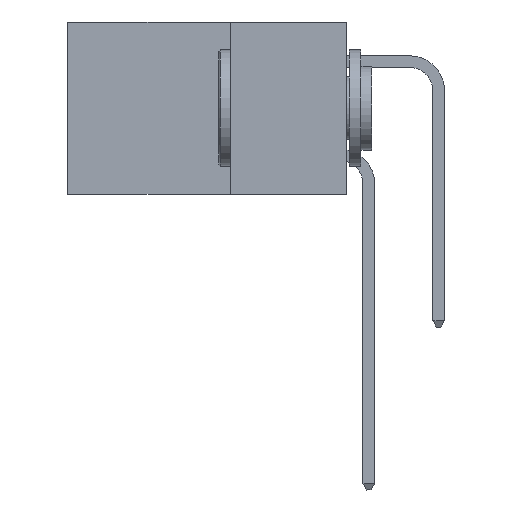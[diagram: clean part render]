
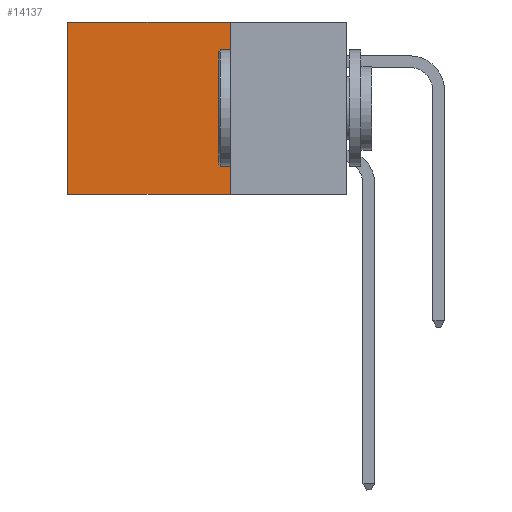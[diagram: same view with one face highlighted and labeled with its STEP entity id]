
A CAD part, left-side view. The second image highlights one B-rep face of the part: STEP entity #14137.
In plain terms, the highlighted planar face has unit normal (-1, 0, 0).
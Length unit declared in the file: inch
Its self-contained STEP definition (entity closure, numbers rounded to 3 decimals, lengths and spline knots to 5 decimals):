
#123 = ORIENTED_EDGE ( 'NONE', *, *, #8447, .T. ) ;
#1247 = VERTEX_POINT ( 'NONE', #9302 ) ;
#1820 = PLANE ( 'NONE',  #14591 ) ;
#2157 = VECTOR ( 'NONE', #8303, 39.37008 ) ;
#2191 = CARTESIAN_POINT ( 'NONE',  ( 0.2875, 0.25, 0. ) ) ;
#2206 = EDGE_LOOP ( 'NONE', ( #123, #6674, #12758, #3878 ) ) ;
#2553 = DIRECTION ( 'NONE',  ( 0., 1., 0. ) ) ;
#3021 = EDGE_CURVE ( 'NONE', #1247, #14370, #9926, .T. ) ;
#3025 = CARTESIAN_POINT ( 'NONE',  ( 0.2875, 0.25, 0. ) ) ;
#3090 = DIRECTION ( 'NONE',  ( 1., 0., 0. ) ) ;
#3215 = LINE ( 'NONE', #9040, #14987 ) ;
#3436 = DIRECTION ( 'NONE',  ( 0., 0., -1. ) ) ;
#3479 = CARTESIAN_POINT ( 'NONE',  ( 0.2875, 0.6, 0. ) ) ;
#3878 = ORIENTED_EDGE ( 'NONE', *, *, #3021, .T. ) ;
#4125 = CARTESIAN_POINT ( 'NONE',  ( 0.2875, 0.25, -0.37 ) ) ;
#5371 = LINE ( 'NONE', #5899, #2157 ) ;
#5899 = CARTESIAN_POINT ( 'NONE',  ( 0.2875, 0.25, -0.37 ) ) ;
#6674 = ORIENTED_EDGE ( 'NONE', *, *, #14986, .F. ) ;
#6804 = CARTESIAN_POINT ( 'NONE',  ( 0.2875, 0.6, -0.37 ) ) ;
#8209 = VECTOR ( 'NONE', #3436, 39.37008 ) ;
#8303 = DIRECTION ( 'NONE',  ( 0., 1., 0. ) ) ;
#8447 = EDGE_CURVE ( 'NONE', #14370, #14822, #3215, .T. ) ;
#8562 = LINE ( 'NONE', #2191, #8209 ) ;
#9000 = CARTESIAN_POINT ( 'NONE',  ( 0.2875, 0.25, 0. ) ) ;
#9040 = CARTESIAN_POINT ( 'NONE',  ( 0.2875, 0.6, 0. ) ) ;
#9302 = CARTESIAN_POINT ( 'NONE',  ( 0.2875, 0.25, 0. ) ) ;
#9543 = VECTOR ( 'NONE', #2553, 39.37008 ) ;
#9926 = LINE ( 'NONE', #3025, #9543 ) ;
#9983 = EDGE_CURVE ( 'NONE', #1247, #13060, #8562, .T. ) ;
#11287 = DIRECTION ( 'NONE',  ( 0., 0., -1. ) ) ;
#12415 = DIRECTION ( 'NONE',  ( 0., 0., -1. ) ) ;
#12758 = ORIENTED_EDGE ( 'NONE', *, *, #9983, .F. ) ;
#13060 = VERTEX_POINT ( 'NONE', #4125 ) ;
#13790 = FACE_OUTER_BOUND ( 'NONE', #2206, .T. ) ;
#14137 = ADVANCED_FACE ( 'NONE', ( #13790 ), #1820, .F. ) ;
#14370 = VERTEX_POINT ( 'NONE', #3479 ) ;
#14591 = AXIS2_PLACEMENT_3D ( 'NONE', #9000, #3090, #11287 ) ;
#14822 = VERTEX_POINT ( 'NONE', #6804 ) ;
#14986 = EDGE_CURVE ( 'NONE', #13060, #14822, #5371, .T. ) ;
#14987 = VECTOR ( 'NONE', #12415, 39.37008 ) ;
